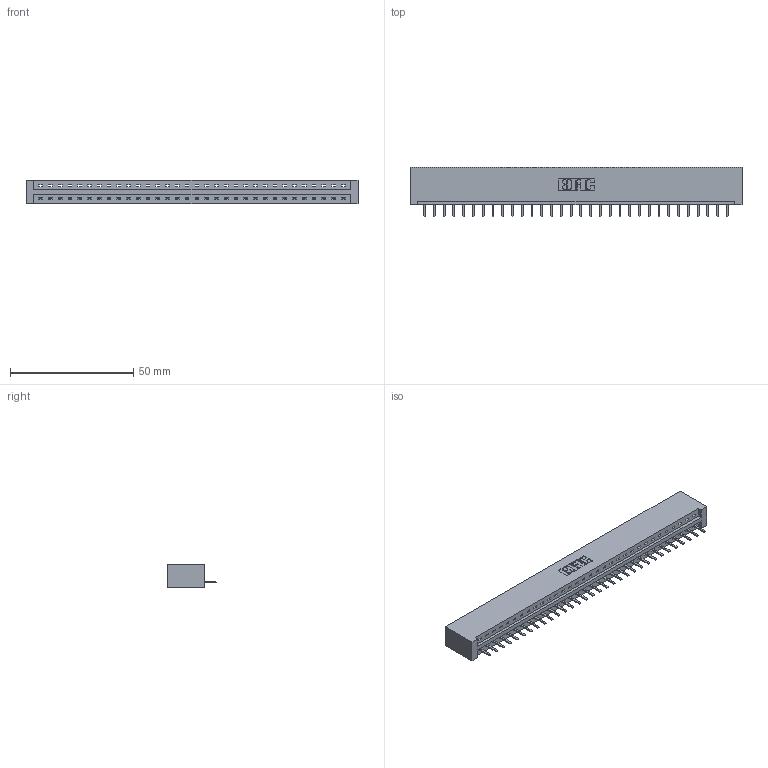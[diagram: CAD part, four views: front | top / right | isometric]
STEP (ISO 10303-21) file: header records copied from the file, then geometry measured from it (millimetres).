
FILE_DESCRIPTION (( 'STEP AP203' ), '1' );
FILE_NAME ('337-032-520-101.STEP', '2019-10-01T02:21:16', ( '' ), ( '' ), 'SwSTEP 2.0', 'SolidWorks 2016', '' );
FILE_SCHEMA (( 'CONFIG_CONTROL_DESIGN' ));
Length unit declared in the file: inch
Products named in the file (3): 337-032-520-101; 337 Part_No Mounting Lugs; 345-292-001_345-293-120
Assembly tree (33 placements, depth 2):
  337-032-520-101
    337 Part_No Mounting Lugs
    345-292-001_345-293-120  x32
Bounding box: 134.67 x 20.02 x 9.4 mm (x, y, z)
Volume: 14518.3 mm3; surface area: 14597.1 mm2
Topology: 33 solids, 33 shells, 2218 faces, 6559 edges, 4286 vertices
Faces by surface type: plane 1602, cylinder 616
Entity records: 24917 total; most frequent: CARTESIAN_POINT 4358, ORIENTED_EDGE 4314, DIRECTION 3669, EDGE_CURVE 2157, VECTOR 2033, LINE 2033, VERTEX_POINT 1434, AXIS2_PLACEMENT_3D 818
